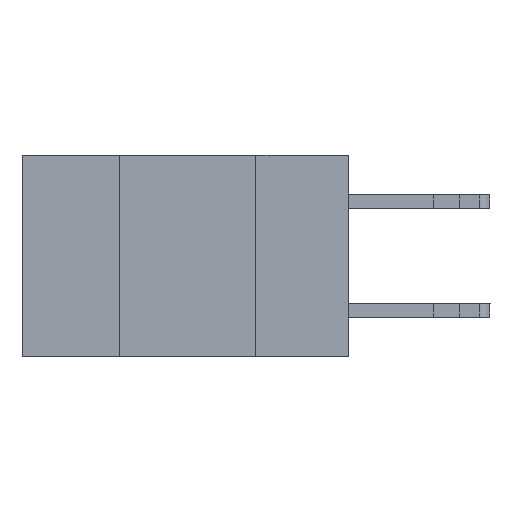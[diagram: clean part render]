
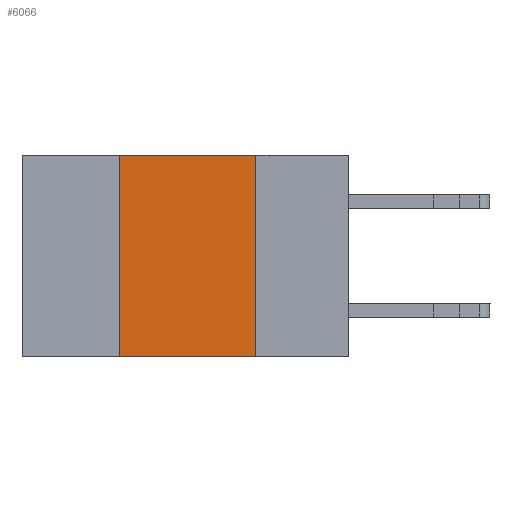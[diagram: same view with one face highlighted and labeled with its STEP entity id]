
A CAD part, left-side view. The second image highlights one B-rep face of the part: STEP entity #6066.
In plain terms, the highlighted planar face has unit normal (-1, 0, 0).
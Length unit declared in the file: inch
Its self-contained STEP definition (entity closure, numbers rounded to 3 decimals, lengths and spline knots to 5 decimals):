
#150 = EDGE_CURVE ( 'NONE', #14240, #5777, #6547, .T. ) ;
#958 = CARTESIAN_POINT ( 'NONE',  ( 0., 0.17, 0. ) ) ;
#2497 = EDGE_CURVE ( 'NONE', #14240, #6819, #21928, .T. ) ;
#3236 = DIRECTION ( 'NONE',  ( 0., -1., 0. ) ) ;
#3719 = ORIENTED_EDGE ( 'NONE', *, *, #5754, .F. ) ;
#3926 = VECTOR ( 'NONE', #25481, 39.37008 ) ;
#4755 = CARTESIAN_POINT ( 'NONE',  ( 0., 0.42, 0. ) ) ;
#5068 = DIRECTION ( 'NONE',  ( 1., 0., 0. ) ) ;
#5334 = CARTESIAN_POINT ( 'NONE',  ( 0., 0.42, 0. ) ) ;
#5754 = EDGE_CURVE ( 'NONE', #6819, #10706, #13008, .T. ) ;
#5777 = VERTEX_POINT ( 'NONE', #11351 ) ;
#6066 = ADVANCED_FACE ( 'NONE', ( #15188 ), #25037, .F. ) ;
#6079 = ORIENTED_EDGE ( 'NONE', *, *, #150, .T. ) ;
#6547 = LINE ( 'NONE', #9838, #23942 ) ;
#6819 = VERTEX_POINT ( 'NONE', #4755 ) ;
#7097 = DIRECTION ( 'NONE',  ( 0., 0., -1. ) ) ;
#7207 = CARTESIAN_POINT ( 'NONE',  ( 0., 0.6, 0. ) ) ;
#7989 = AXIS2_PLACEMENT_3D ( 'NONE', #16991, #5068, #7097 ) ;
#8251 = DIRECTION ( 'NONE',  ( 0., 0., -1. ) ) ;
#9838 = CARTESIAN_POINT ( 'NONE',  ( 0., 0.6, -0.37 ) ) ;
#9919 = DIRECTION ( 'NONE',  ( 0., -1., 0. ) ) ;
#10381 = VECTOR ( 'NONE', #3236, 39.37008 ) ;
#10706 = VERTEX_POINT ( 'NONE', #958 ) ;
#11351 = CARTESIAN_POINT ( 'NONE',  ( 0., 0.17, -0.37 ) ) ;
#12256 = CARTESIAN_POINT ( 'NONE',  ( 0., 0.17, 0. ) ) ;
#12291 = EDGE_CURVE ( 'NONE', #10706, #5777, #23441, .T. ) ;
#13008 = LINE ( 'NONE', #7207, #10381 ) ;
#14240 = VERTEX_POINT ( 'NONE', #15717 ) ;
#14986 = EDGE_LOOP ( 'NONE', ( #18471, #3719, #22400, #6079 ) ) ;
#15188 = FACE_OUTER_BOUND ( 'NONE', #14986, .T. ) ;
#15717 = CARTESIAN_POINT ( 'NONE',  ( 0., 0.42, -0.37 ) ) ;
#16991 = CARTESIAN_POINT ( 'NONE',  ( 0., 0.6, 0. ) ) ;
#18471 = ORIENTED_EDGE ( 'NONE', *, *, #12291, .F. ) ;
#21928 = LINE ( 'NONE', #5334, #3926 ) ;
#22400 = ORIENTED_EDGE ( 'NONE', *, *, #2497, .F. ) ;
#23441 = LINE ( 'NONE', #12256, #25928 ) ;
#23942 = VECTOR ( 'NONE', #9919, 39.37008 ) ;
#25037 = PLANE ( 'NONE',  #7989 ) ;
#25481 = DIRECTION ( 'NONE',  ( 0., 0., 1. ) ) ;
#25928 = VECTOR ( 'NONE', #8251, 39.37008 ) ;
